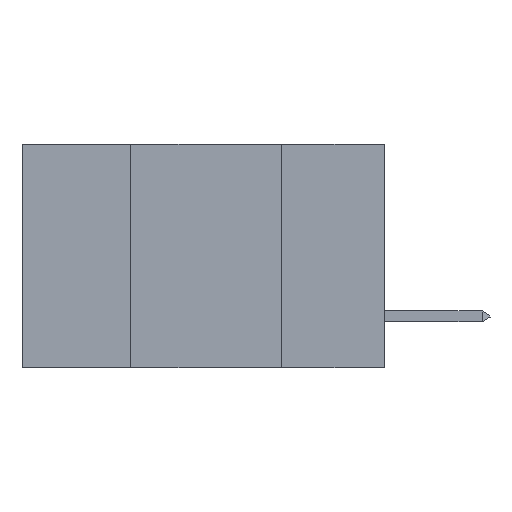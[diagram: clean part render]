
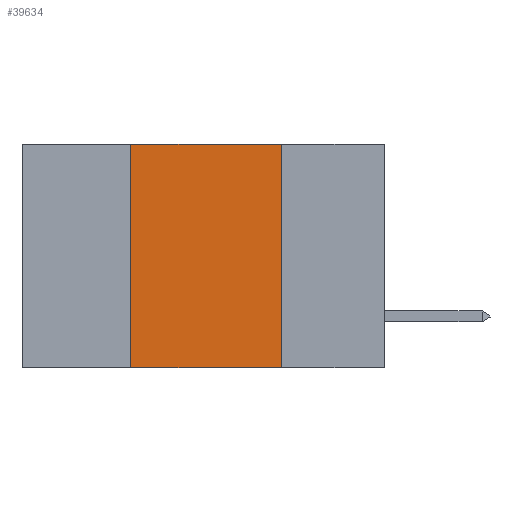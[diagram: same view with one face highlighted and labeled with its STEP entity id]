
A CAD part, left-side view. The second image highlights one B-rep face of the part: STEP entity #39634.
In plain terms, the highlighted planar face has unit normal (-1, 0, 0).
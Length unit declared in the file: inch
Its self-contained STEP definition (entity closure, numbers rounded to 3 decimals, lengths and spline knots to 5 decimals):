
#2147 = CARTESIAN_POINT ( 'NONE',  ( 0., 0.17, 0. ) ) ;
#2828 = EDGE_CURVE ( 'NONE', #36098, #45684, #13650, .T. ) ;
#3908 = EDGE_CURVE ( 'NONE', #18853, #36098, #29188, .T. ) ;
#5074 = VECTOR ( 'NONE', #29203, 39.37008 ) ;
#6255 = VECTOR ( 'NONE', #36720, 39.37008 ) ;
#6776 = VERTEX_POINT ( 'NONE', #18601 ) ;
#7531 = PLANE ( 'NONE',  #24695 ) ;
#10835 = FACE_OUTER_BOUND ( 'NONE', #24287, .T. ) ;
#13154 = ORIENTED_EDGE ( 'NONE', *, *, #2828, .F. ) ;
#13650 = LINE ( 'NONE', #21274, #5074 ) ;
#15211 = CARTESIAN_POINT ( 'NONE',  ( 0., 0.42, 0. ) ) ;
#18079 = CARTESIAN_POINT ( 'NONE',  ( 0., 0.42, 0. ) ) ;
#18601 = CARTESIAN_POINT ( 'NONE',  ( 0., 0.17, -0.37 ) ) ;
#18678 = VECTOR ( 'NONE', #49523, 39.37008 ) ;
#18718 = CARTESIAN_POINT ( 'NONE',  ( 0., 0.6, 0. ) ) ;
#18853 = VERTEX_POINT ( 'NONE', #19570 ) ;
#18898 = DIRECTION ( 'NONE',  ( 0., 0., -1. ) ) ;
#19570 = CARTESIAN_POINT ( 'NONE',  ( 0., 0.42, -0.37 ) ) ;
#20218 = LINE ( 'NONE', #20570, #20829 ) ;
#20570 = CARTESIAN_POINT ( 'NONE',  ( 0., 0.6, -0.37 ) ) ;
#20829 = VECTOR ( 'NONE', #26676, 39.37008 ) ;
#21274 = CARTESIAN_POINT ( 'NONE',  ( 0., 0.6, 0. ) ) ;
#24287 = EDGE_LOOP ( 'NONE', ( #49546, #13154, #27071, #35343 ) ) ;
#24695 = AXIS2_PLACEMENT_3D ( 'NONE', #18718, #50480, #18898 ) ;
#25078 = EDGE_CURVE ( 'NONE', #45684, #6776, #49293, .T. ) ;
#26676 = DIRECTION ( 'NONE',  ( 0., -1., 0. ) ) ;
#27071 = ORIENTED_EDGE ( 'NONE', *, *, #3908, .F. ) ;
#29188 = LINE ( 'NONE', #18079, #18678 ) ;
#29203 = DIRECTION ( 'NONE',  ( 0., -1., 0. ) ) ;
#32227 = EDGE_CURVE ( 'NONE', #18853, #6776, #20218, .T. ) ;
#35343 = ORIENTED_EDGE ( 'NONE', *, *, #32227, .T. ) ;
#35397 = CARTESIAN_POINT ( 'NONE',  ( 0., 0.17, 0. ) ) ;
#36098 = VERTEX_POINT ( 'NONE', #15211 ) ;
#36720 = DIRECTION ( 'NONE',  ( 0., 0., -1. ) ) ;
#39634 = ADVANCED_FACE ( 'NONE', ( #10835 ), #7531, .F. ) ;
#45684 = VERTEX_POINT ( 'NONE', #35397 ) ;
#49293 = LINE ( 'NONE', #2147, #6255 ) ;
#49523 = DIRECTION ( 'NONE',  ( 0., 0., 1. ) ) ;
#49546 = ORIENTED_EDGE ( 'NONE', *, *, #25078, .F. ) ;
#50480 = DIRECTION ( 'NONE',  ( 1., 0., 0. ) ) ;
